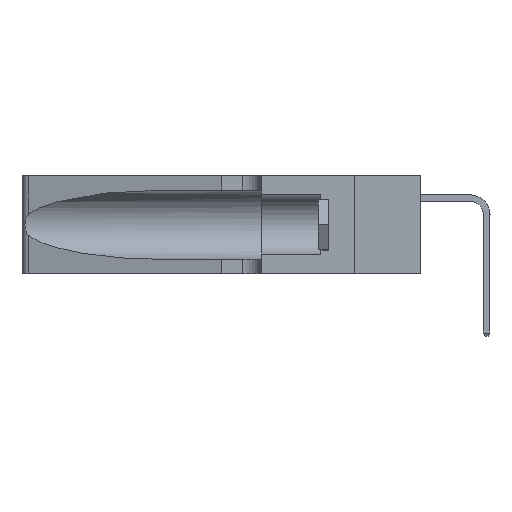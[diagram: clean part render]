
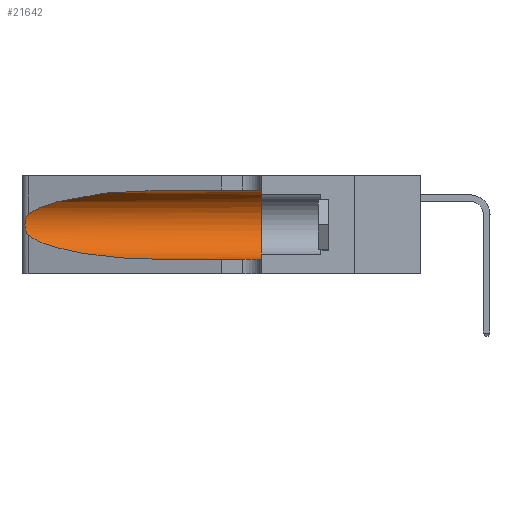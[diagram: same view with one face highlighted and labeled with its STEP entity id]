
A CAD part, left-side view. The second image highlights one B-rep face of the part: STEP entity #21642.
In plain terms, the highlighted cylindrical face has radius 3.308 mm (diameter 6.617 mm), a partial arc.
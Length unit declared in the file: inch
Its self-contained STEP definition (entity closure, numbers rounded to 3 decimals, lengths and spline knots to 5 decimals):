
#172 = B_SPLINE_CURVE_WITH_KNOTS ( 'NONE', 3,
 ( #32264, #4864, #12843, #40081, #16798, #43937, #20715, #47836, #24644, #1079, #28538, #5041, #32441, #9008 ),
 .UNSPECIFIED., .F., .F.,
 ( 4, 2, 2, 2, 2, 2, 4 ),
 ( 0., 0.00027, 0.00053, 0.00107, 0.0016, 0.00187, 0.00214 ),
 .UNSPECIFIED. ) ;
#343 = CARTESIAN_POINT ( 'NONE',  ( 0.25487, 1.22718, 0.22369 ) ) ;
#1079 = CARTESIAN_POINT ( 'NONE',  ( 0.25856, 1.23593, 0.16098 ) ) ;
#1125 = ORIENTED_EDGE ( 'NONE', *, *, #25680, .T. ) ;
#1230 =( BOUNDED_CURVE ( )  B_SPLINE_CURVE ( 3, ( #25988, #49142, #6408, #33786 ),
 .UNSPECIFIED., .F., .T. ) 
 B_SPLINE_CURVE_WITH_KNOTS ( ( 4, 4 ),
 ( 3.44316, 4.71239 ),
 .UNSPECIFIED. ) 
 CURVE ( )  GEOMETRIC_REPRESENTATION_ITEM ( )  RATIONAL_B_SPLINE_CURVE ( ( 1., 0.87, 0.87, 1. ) ) 
 REPRESENTATION_ITEM ( '' )  );
#1509 = EDGE_LOOP ( 'NONE', ( #1125, #5953, #16313, #26194, #29750, #24485 ) ) ;
#1745 =( BOUNDED_CURVE ( )  B_SPLINE_CURVE ( 3, ( #23922, #19987, #31559, #343 ),
 .UNSPECIFIED., .F., .F. ) 
 B_SPLINE_CURVE_WITH_KNOTS ( ( 4, 4 ),
 ( 1.5708, 2.84003 ),
 .UNSPECIFIED. ) 
 CURVE ( )  GEOMETRIC_REPRESENTATION_ITEM ( )  RATIONAL_B_SPLINE_CURVE ( ( 1., 0.87, 0.87, 1. ) ) 
 REPRESENTATION_ITEM ( '' )  );
#2066 = CARTESIAN_POINT ( 'NONE',  ( 0.1305, 1.61858, 0.31525 ) ) ;
#2622 = EDGE_CURVE ( 'NONE', #26095, #11094, #9844, .T. ) ;
#2894 = CARTESIAN_POINT ( 'NONE',  ( 0.1305, 0.72297, 0.31525 ) ) ;
#3880 = VERTEX_POINT ( 'NONE', #45282 ) ;
#4588 = VERTEX_POINT ( 'NONE', #36802 ) ;
#4864 = CARTESIAN_POINT ( 'NONE',  ( 0.25555, 1.22994, 0.2215 ) ) ;
#5041 = CARTESIAN_POINT ( 'NONE',  ( 0.25639, 1.23186, 0.15144 ) ) ;
#5953 = ORIENTED_EDGE ( 'NONE', *, *, #36951, .T. ) ;
#6003 = DIRECTION ( 'NONE',  ( 0., -1., 0. ) ) ;
#6408 = CARTESIAN_POINT ( 'NONE',  ( 0.18966, 0.96281, 0.05475 ) ) ;
#6786 = FACE_OUTER_BOUND ( 'NONE', #1509, .T. ) ;
#7270 = LINE ( 'NONE', #41266, #28139 ) ;
#7383 = VECTOR ( 'NONE', #6003, 39.37008 ) ;
#9008 = CARTESIAN_POINT ( 'NONE',  ( 0.25487, 1.22718, 0.14631 ) ) ;
#9312 = CARTESIAN_POINT ( 'NONE',  ( 0.1305, 0.35, 0.185 ) ) ;
#9844 = LINE ( 'NONE', #2066, #7383 ) ;
#10533 = AXIS2_PLACEMENT_3D ( 'NONE', #47743, #20625, #12740 ) ;
#11094 = VERTEX_POINT ( 'NONE', #43819 ) ;
#12740 = DIRECTION ( 'NONE',  ( 0., 0., -1. ) ) ;
#12843 = CARTESIAN_POINT ( 'NONE',  ( 0.25639, 1.23184, 0.21858 ) ) ;
#13317 = DIRECTION ( 'NONE',  ( 0., 0., 1. ) ) ;
#16068 = CYLINDRICAL_SURFACE ( 'NONE', #10533, 0.13025 ) ;
#16313 = ORIENTED_EDGE ( 'NONE', *, *, #30417, .T. ) ;
#16798 = CARTESIAN_POINT ( 'NONE',  ( 0.25854, 1.2359, 0.20912 ) ) ;
#17538 = EDGE_CURVE ( 'NONE', #11094, #4588, #20111, .T. ) ;
#19079 = VERTEX_POINT ( 'NONE', #38885 ) ;
#19404 = CARTESIAN_POINT ( 'NONE',  ( 0.25487, 1.22718, 0.22369 ) ) ;
#19987 = CARTESIAN_POINT ( 'NONE',  ( 0.18966, 0.96281, 0.31525 ) ) ;
#20111 = CIRCLE ( 'NONE', #23281, 0.13025 ) ;
#20625 = DIRECTION ( 'NONE',  ( 0., -1., 0. ) ) ;
#20715 = CARTESIAN_POINT ( 'NONE',  ( 0.26075, 1.23896, 0.19203 ) ) ;
#21642 = ADVANCED_FACE ( 'NONE', ( #6786 ), #16068, .F. ) ;
#23281 = AXIS2_PLACEMENT_3D ( 'NONE', #9312, #36669, #13317 ) ;
#23922 = CARTESIAN_POINT ( 'NONE',  ( 0.1305, 0.72297, 0.31525 ) ) ;
#24485 = ORIENTED_EDGE ( 'NONE', *, *, #2622, .F. ) ;
#24644 = CARTESIAN_POINT ( 'NONE',  ( 0.26017, 1.23833, 0.17102 ) ) ;
#25680 = EDGE_CURVE ( 'NONE', #26095, #43229, #1745, .T. ) ;
#25988 = CARTESIAN_POINT ( 'NONE',  ( 0.25487, 1.22718, 0.14631 ) ) ;
#26095 = VERTEX_POINT ( 'NONE', #2894 ) ;
#26194 = ORIENTED_EDGE ( 'NONE', *, *, #39027, .T. ) ;
#28139 = VECTOR ( 'NONE', #44925, 39.37008 ) ;
#28538 = CARTESIAN_POINT ( 'NONE',  ( 0.25789, 1.23486, 0.15765 ) ) ;
#29750 = ORIENTED_EDGE ( 'NONE', *, *, #17538, .F. ) ;
#30417 = EDGE_CURVE ( 'NONE', #19079, #3880, #1230, .T. ) ;
#31559 = CARTESIAN_POINT ( 'NONE',  ( 0.2373, 1.15595, 0.28018 ) ) ;
#32264 = CARTESIAN_POINT ( 'NONE',  ( 0.25487, 1.22718, 0.22369 ) ) ;
#32441 = CARTESIAN_POINT ( 'NONE',  ( 0.25555, 1.22993, 0.14849 ) ) ;
#33786 = CARTESIAN_POINT ( 'NONE',  ( 0.1305, 0.72297, 0.05475 ) ) ;
#36669 = DIRECTION ( 'NONE',  ( 0., 1., 0. ) ) ;
#36802 = CARTESIAN_POINT ( 'NONE',  ( 0.1305, 0.35, 0.05475 ) ) ;
#36951 = EDGE_CURVE ( 'NONE', #43229, #19079, #172, .T. ) ;
#38885 = CARTESIAN_POINT ( 'NONE',  ( 0.25487, 1.22718, 0.14631 ) ) ;
#39027 = EDGE_CURVE ( 'NONE', #3880, #4588, #7270, .T. ) ;
#40081 = CARTESIAN_POINT ( 'NONE',  ( 0.25787, 1.23484, 0.2124 ) ) ;
#41266 = CARTESIAN_POINT ( 'NONE',  ( 0.1305, 1.61858, 0.05475 ) ) ;
#43229 = VERTEX_POINT ( 'NONE', #19404 ) ;
#43819 = CARTESIAN_POINT ( 'NONE',  ( 0.1305, 0.35, 0.31525 ) ) ;
#43937 = CARTESIAN_POINT ( 'NONE',  ( 0.26018, 1.23835, 0.19895 ) ) ;
#44925 = DIRECTION ( 'NONE',  ( 0., -1., 0. ) ) ;
#45282 = CARTESIAN_POINT ( 'NONE',  ( 0.1305, 0.72297, 0.05475 ) ) ;
#47743 = CARTESIAN_POINT ( 'NONE',  ( 0.1305, 1.61858, 0.185 ) ) ;
#47836 = CARTESIAN_POINT ( 'NONE',  ( 0.26075, 1.23896, 0.178 ) ) ;
#49142 = CARTESIAN_POINT ( 'NONE',  ( 0.2373, 1.15595, 0.08982 ) ) ;
